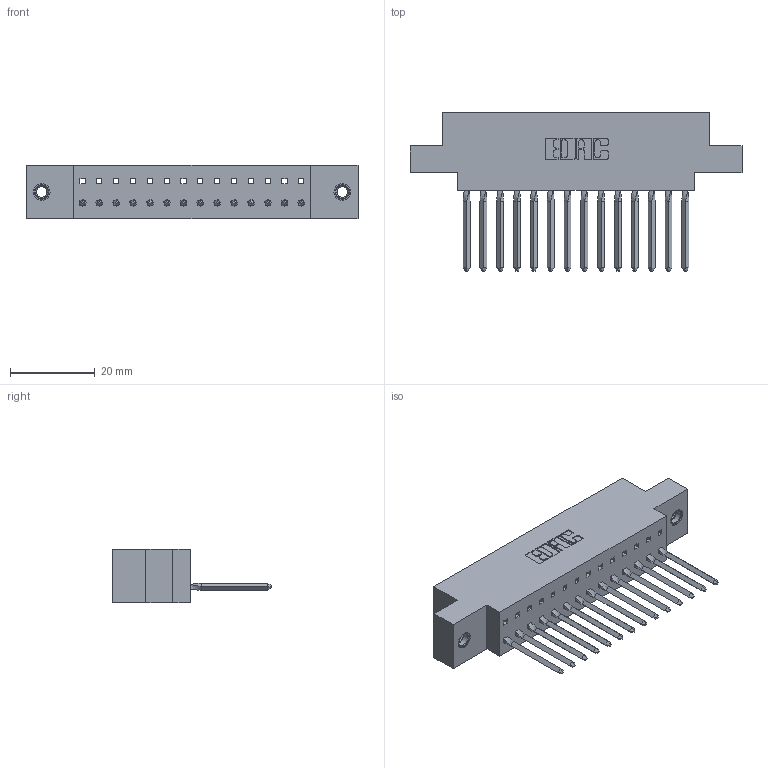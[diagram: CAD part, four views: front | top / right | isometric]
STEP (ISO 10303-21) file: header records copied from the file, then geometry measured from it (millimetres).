
FILE_DESCRIPTION (( 'STEP AP203' ), '1' );
FILE_NAME ('317-014-542-607.STEP', '2020-02-27T14:32:34', ( '' ), ( '' ), 'SwSTEP 2.0', 'SolidWorks 2016', '' );
FILE_SCHEMA (( 'CONFIG_CONTROL_DESIGN' ));
Length unit declared in the file: inch
Products named in the file (4): 317-014-542-607; 345-250-001_345-250-005-103; 317 Part_.156 Dia - TI; 317-290-003_542
Assembly tree (17 placements, depth 2):
  317-014-542-607
    317 Part_.156 Dia - TI
    317-290-003_542  x14
    345-250-001_345-250-005-103  x2
Bounding box: 78.18 x 37.34 x 12.7 mm (x, y, z)
Volume: 11318.9 mm3; surface area: 13216.1 mm2
Topology: 17 solids, 17 shells, 1212 faces, 3449 edges, 2226 vertices
Faces by surface type: plane 986, cylinder 154, bspline 56, cone 12, torus 4
Entity records: 23898 total; most frequent: CARTESIAN_POINT 4450, ORIENTED_EDGE 4120, DIRECTION 3526, EDGE_CURVE 2060, LINE 1870, VECTOR 1870, VERTEX_POINT 1364, AXIS2_PLACEMENT_3D 828
